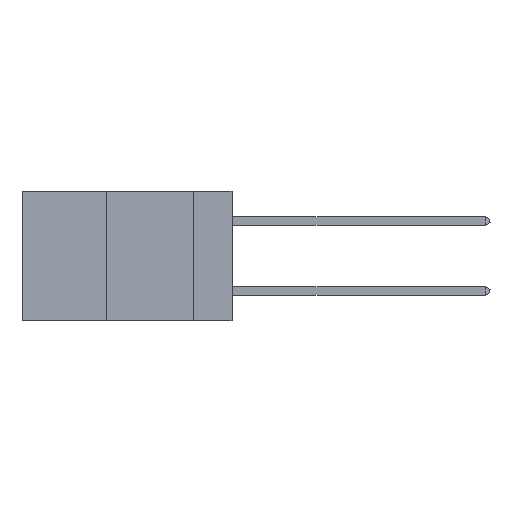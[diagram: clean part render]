
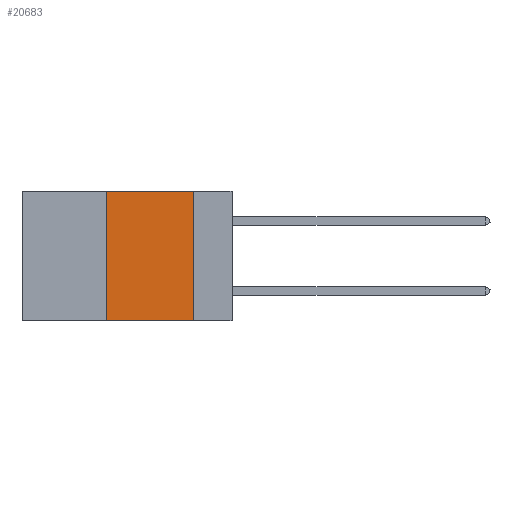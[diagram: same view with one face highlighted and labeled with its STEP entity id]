
A CAD part, left-side view. The second image highlights one B-rep face of the part: STEP entity #20683.
In plain terms, the highlighted planar face has unit normal (-1, 0, 0).
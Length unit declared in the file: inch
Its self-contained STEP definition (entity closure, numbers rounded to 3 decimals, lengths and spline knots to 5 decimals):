
#335 = CARTESIAN_POINT ( 'NONE',  ( 0., 0.36, 0. ) ) ;
#431 = CARTESIAN_POINT ( 'NONE',  ( 0., 0.36, -0.37 ) ) ;
#1441 = EDGE_LOOP ( 'NONE', ( #13864, #18688, #29271, #4557 ) ) ;
#2503 = VECTOR ( 'NONE', #25804, 39.37008 ) ;
#3756 = LINE ( 'NONE', #23546, #15115 ) ;
#4047 = DIRECTION ( 'NONE',  ( 0., 0., -1. ) ) ;
#4557 = ORIENTED_EDGE ( 'NONE', *, *, #14037, .T. ) ;
#4791 = LINE ( 'NONE', #8062, #22505 ) ;
#5395 = VERTEX_POINT ( 'NONE', #431 ) ;
#5445 = CARTESIAN_POINT ( 'NONE',  ( 0., 0.6, 0. ) ) ;
#5553 = DIRECTION ( 'NONE',  ( 0., 0., -1. ) ) ;
#6718 = DIRECTION ( 'NONE',  ( 0., -1., 0. ) ) ;
#8062 = CARTESIAN_POINT ( 'NONE',  ( 0., 0.36, 0. ) ) ;
#8122 = EDGE_CURVE ( 'NONE', #5395, #10809, #4791, .T. ) ;
#9024 = CARTESIAN_POINT ( 'NONE',  ( 0., 0.6, 0. ) ) ;
#10626 = CARTESIAN_POINT ( 'NONE',  ( 0., 0.11, 0. ) ) ;
#10809 = VERTEX_POINT ( 'NONE', #335 ) ;
#11489 = AXIS2_PLACEMENT_3D ( 'NONE', #5445, #19987, #5553 ) ;
#12556 = VERTEX_POINT ( 'NONE', #10626 ) ;
#13683 = CARTESIAN_POINT ( 'NONE',  ( 0., 0.11, 0. ) ) ;
#13864 = ORIENTED_EDGE ( 'NONE', *, *, #14630, .F. ) ;
#14037 = EDGE_CURVE ( 'NONE', #5395, #18819, #3756, .T. ) ;
#14630 = EDGE_CURVE ( 'NONE', #12556, #18819, #18437, .T. ) ;
#15115 = VECTOR ( 'NONE', #6718, 39.37008 ) ;
#15196 = PLANE ( 'NONE',  #11489 ) ;
#15236 = EDGE_CURVE ( 'NONE', #10809, #12556, #26602, .T. ) ;
#15391 = DIRECTION ( 'NONE',  ( 0., 0., 1. ) ) ;
#18437 = LINE ( 'NONE', #13683, #23294 ) ;
#18688 = ORIENTED_EDGE ( 'NONE', *, *, #15236, .F. ) ;
#18819 = VERTEX_POINT ( 'NONE', #20194 ) ;
#19962 = FACE_OUTER_BOUND ( 'NONE', #1441, .T. ) ;
#19987 = DIRECTION ( 'NONE',  ( 1., 0., 0. ) ) ;
#20194 = CARTESIAN_POINT ( 'NONE',  ( 0., 0.11, -0.37 ) ) ;
#20683 = ADVANCED_FACE ( 'NONE', ( #19962 ), #15196, .F. ) ;
#22505 = VECTOR ( 'NONE', #15391, 39.37008 ) ;
#23294 = VECTOR ( 'NONE', #4047, 39.37008 ) ;
#23546 = CARTESIAN_POINT ( 'NONE',  ( 0., 0.6, -0.37 ) ) ;
#25804 = DIRECTION ( 'NONE',  ( 0., -1., 0. ) ) ;
#26602 = LINE ( 'NONE', #9024, #2503 ) ;
#29271 = ORIENTED_EDGE ( 'NONE', *, *, #8122, .F. ) ;
